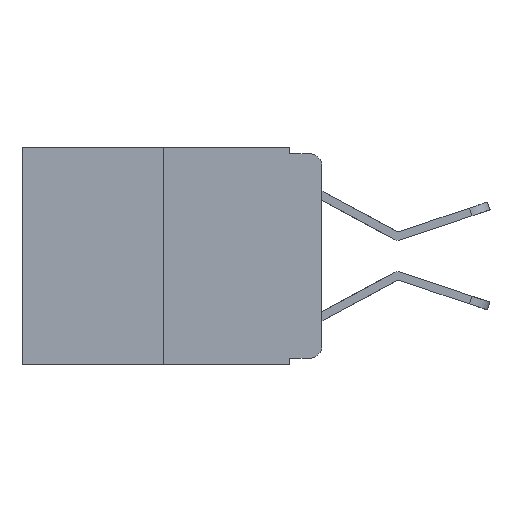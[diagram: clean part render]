
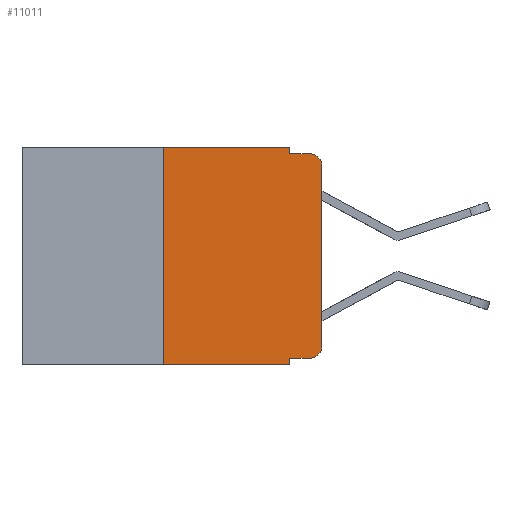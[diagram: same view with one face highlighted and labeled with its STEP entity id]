
A CAD part, left-side view. The second image highlights one B-rep face of the part: STEP entity #11011.
In plain terms, the highlighted planar face has unit normal (-1, 0, 0).
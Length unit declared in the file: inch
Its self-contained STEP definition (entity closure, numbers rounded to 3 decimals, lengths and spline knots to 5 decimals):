
#170 = EDGE_CURVE ( 'NONE', #5191, #3026, #13107, .T. ) ;
#272 = VERTEX_POINT ( 'NONE', #7629 ) ;
#435 = DIRECTION ( 'NONE',  ( 0., -1., 0. ) ) ;
#735 = PLANE ( 'NONE',  #13123 ) ;
#771 = VECTOR ( 'NONE', #4463, 39.37008 ) ;
#1055 = EDGE_CURVE ( 'NONE', #12489, #3026, #1737, .T. ) ;
#1406 = CARTESIAN_POINT ( 'NONE',  ( 0., 0.02, -0.313 ) ) ;
#1505 = ORIENTED_EDGE ( 'NONE', *, *, #14300, .F. ) ;
#1560 = VECTOR ( 'NONE', #9990, 39.37008 ) ;
#1737 = CIRCLE ( 'NONE', #13883, 0.02 ) ;
#1783 = DIRECTION ( 'NONE',  ( 0., 0., 1. ) ) ;
#1832 = EDGE_CURVE ( 'NONE', #272, #9620, #7709, .T. ) ;
#1930 = EDGE_CURVE ( 'NONE', #5596, #12489, #9371, .T. ) ;
#2027 = DIRECTION ( 'NONE',  ( 1., 0., 0. ) ) ;
#2071 = ORIENTED_EDGE ( 'NONE', *, *, #15083, .F. ) ;
#2496 = CARTESIAN_POINT ( 'NONE',  ( 0., 0.051, 0. ) ) ;
#2664 = DIRECTION ( 'NONE',  ( 0., 0., -1. ) ) ;
#3026 = VERTEX_POINT ( 'NONE', #13436 ) ;
#3328 = LINE ( 'NONE', #8226, #15638 ) ;
#3437 = DIRECTION ( 'NONE',  ( 0., 0., 1. ) ) ;
#3522 = CARTESIAN_POINT ( 'NONE',  ( 0., 0.051, -0.333 ) ) ;
#3538 = VECTOR ( 'NONE', #5663, 39.37008 ) ;
#3887 = DIRECTION ( 'NONE',  ( -1., 0., 0. ) ) ;
#3927 = LINE ( 'NONE', #4492, #3538 ) ;
#3928 = CARTESIAN_POINT ( 'NONE',  ( 0., 0.02, -0.03 ) ) ;
#4026 = LINE ( 'NONE', #11405, #10402 ) ;
#4463 = DIRECTION ( 'NONE',  ( 0., -1., 0. ) ) ;
#4474 = CARTESIAN_POINT ( 'NONE',  ( 0., 0., -0.313 ) ) ;
#4492 = CARTESIAN_POINT ( 'NONE',  ( 0., 0.051, 0. ) ) ;
#4607 = LINE ( 'NONE', #9026, #10974 ) ;
#4631 = VERTEX_POINT ( 'NONE', #3522 ) ;
#4724 = CARTESIAN_POINT ( 'NONE',  ( 0., 0., 0. ) ) ;
#4942 = EDGE_CURVE ( 'NONE', #6660, #5151, #4026, .T. ) ;
#4975 = ORIENTED_EDGE ( 'NONE', *, *, #170, .F. ) ;
#5151 = VERTEX_POINT ( 'NONE', #15309 ) ;
#5191 = VERTEX_POINT ( 'NONE', #14230 ) ;
#5406 = DIRECTION ( 'NONE',  ( 0., -1., 0. ) ) ;
#5561 = ORIENTED_EDGE ( 'NONE', *, *, #11958, .T. ) ;
#5596 = VERTEX_POINT ( 'NONE', #4474 ) ;
#5663 = DIRECTION ( 'NONE',  ( 0., 0., -1. ) ) ;
#5816 = VECTOR ( 'NONE', #1783, 39.37008 ) ;
#6660 = VERTEX_POINT ( 'NONE', #9936 ) ;
#7235 = ORIENTED_EDGE ( 'NONE', *, *, #1832, .F. ) ;
#7629 = CARTESIAN_POINT ( 'NONE',  ( 0., 0.25, 0. ) ) ;
#7709 = LINE ( 'NONE', #11499, #771 ) ;
#8226 = CARTESIAN_POINT ( 'NONE',  ( 0., 0.25, 0. ) ) ;
#8433 = CARTESIAN_POINT ( 'NONE',  ( 0., 0., -0.03 ) ) ;
#8448 = DIRECTION ( 'NONE',  ( 0., -1., 0. ) ) ;
#9026 = CARTESIAN_POINT ( 'NONE',  ( 0., 0.051, -0.333 ) ) ;
#9236 = CARTESIAN_POINT ( 'NONE',  ( 0., 0.473, 0. ) ) ;
#9371 = LINE ( 'NONE', #4724, #5816 ) ;
#9620 = VERTEX_POINT ( 'NONE', #2496 ) ;
#9868 = DIRECTION ( 'NONE',  ( -1., 0., 0. ) ) ;
#9888 = VECTOR ( 'NONE', #8448, 39.37008 ) ;
#9936 = CARTESIAN_POINT ( 'NONE',  ( 0., 0.25, -0.343 ) ) ;
#9990 = DIRECTION ( 'NONE',  ( 0., 0., -1. ) ) ;
#10402 = VECTOR ( 'NONE', #5406, 39.37008 ) ;
#10418 = VERTEX_POINT ( 'NONE', #14043 ) ;
#10487 = DIRECTION ( 'NONE',  ( 0., 0., -1. ) ) ;
#10974 = VECTOR ( 'NONE', #435, 39.37008 ) ;
#11011 = ADVANCED_FACE ( 'NONE', ( #14544 ), #735, .F. ) ;
#11207 = CARTESIAN_POINT ( 'NONE',  ( 0., 0.051, 0. ) ) ;
#11405 = CARTESIAN_POINT ( 'NONE',  ( 0., 0.473, -0.343 ) ) ;
#11499 = CARTESIAN_POINT ( 'NONE',  ( 0., 0.473, 0. ) ) ;
#11703 = EDGE_LOOP ( 'NONE', ( #15001, #13748, #4975, #2071, #7235, #1505, #14486, #12872, #13247, #5561 ) ) ;
#11958 = EDGE_CURVE ( 'NONE', #10418, #5596, #14891, .T. ) ;
#12489 = VERTEX_POINT ( 'NONE', #8433 ) ;
#12770 = EDGE_CURVE ( 'NONE', #4631, #10418, #4607, .T. ) ;
#12872 = ORIENTED_EDGE ( 'NONE', *, *, #13560, .F. ) ;
#13107 = LINE ( 'NONE', #13277, #9888 ) ;
#13123 = AXIS2_PLACEMENT_3D ( 'NONE', #9236, #2027, #10487 ) ;
#13247 = ORIENTED_EDGE ( 'NONE', *, *, #12770, .T. ) ;
#13277 = CARTESIAN_POINT ( 'NONE',  ( 0., 0.051, -0.01 ) ) ;
#13436 = CARTESIAN_POINT ( 'NONE',  ( 0., 0.02, -0.01 ) ) ;
#13560 = EDGE_CURVE ( 'NONE', #4631, #5151, #3927, .T. ) ;
#13748 = ORIENTED_EDGE ( 'NONE', *, *, #1055, .T. ) ;
#13883 = AXIS2_PLACEMENT_3D ( 'NONE', #3928, #3887, #14207 ) ;
#14043 = CARTESIAN_POINT ( 'NONE',  ( 0., 0.02, -0.333 ) ) ;
#14207 = DIRECTION ( 'NONE',  ( 0., 0., -1. ) ) ;
#14230 = CARTESIAN_POINT ( 'NONE',  ( 0., 0.051, -0.01 ) ) ;
#14300 = EDGE_CURVE ( 'NONE', #6660, #272, #3328, .T. ) ;
#14340 = LINE ( 'NONE', #11207, #1560 ) ;
#14486 = ORIENTED_EDGE ( 'NONE', *, *, #4942, .T. ) ;
#14544 = FACE_OUTER_BOUND ( 'NONE', #11703, .T. ) ;
#14574 = AXIS2_PLACEMENT_3D ( 'NONE', #1406, #9868, #2664 ) ;
#14891 = CIRCLE ( 'NONE', #14574, 0.02 ) ;
#15001 = ORIENTED_EDGE ( 'NONE', *, *, #1930, .T. ) ;
#15083 = EDGE_CURVE ( 'NONE', #9620, #5191, #14340, .T. ) ;
#15309 = CARTESIAN_POINT ( 'NONE',  ( 0., 0.051, -0.343 ) ) ;
#15638 = VECTOR ( 'NONE', #3437, 39.37008 ) ;
